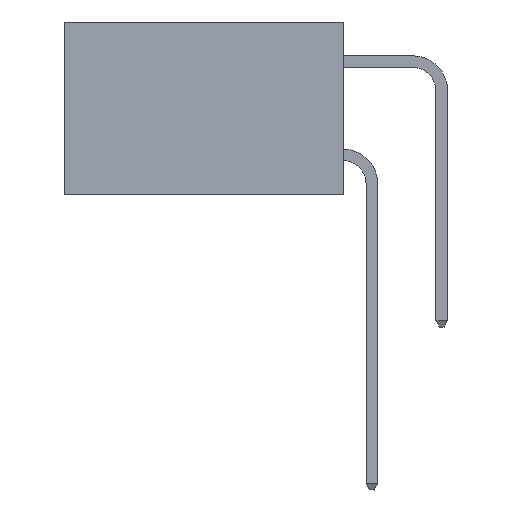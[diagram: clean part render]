
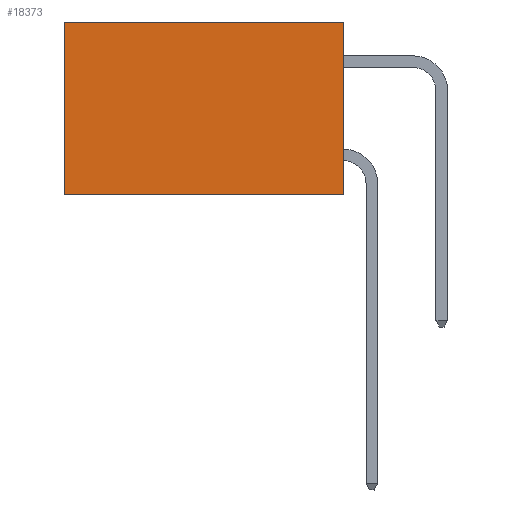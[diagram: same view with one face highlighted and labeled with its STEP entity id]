
A CAD part, left-side view. The second image highlights one B-rep face of the part: STEP entity #18373.
In plain terms, the highlighted planar face has unit normal (-1, 0, 0).
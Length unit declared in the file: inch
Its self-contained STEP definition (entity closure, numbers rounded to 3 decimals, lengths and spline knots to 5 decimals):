
#243 = VERTEX_POINT ( 'NONE', #23693 ) ;
#539 = ORIENTED_EDGE ( 'NONE', *, *, #4084, .T. ) ;
#1354 = LINE ( 'NONE', #24016, #4735 ) ;
#1609 = LINE ( 'NONE', #6266, #12739 ) ;
#3948 = CARTESIAN_POINT ( 'NONE',  ( 0.298, 0.6, 0. ) ) ;
#4084 = EDGE_CURVE ( 'NONE', #29952, #25502, #1609, .T. ) ;
#4362 = DIRECTION ( 'NONE',  ( 0., 0., -1. ) ) ;
#4735 = VECTOR ( 'NONE', #11901, 39.37008 ) ;
#5159 = CARTESIAN_POINT ( 'NONE',  ( 0.298, 0., 0. ) ) ;
#5427 = DIRECTION ( 'NONE',  ( 0., 0., -1. ) ) ;
#5473 = LINE ( 'NONE', #3948, #22225 ) ;
#6266 = CARTESIAN_POINT ( 'NONE',  ( 0.298, 0., 0. ) ) ;
#7708 = CARTESIAN_POINT ( 'NONE',  ( 0.298, 0., -0.37 ) ) ;
#9049 = EDGE_CURVE ( 'NONE', #25502, #29524, #5473, .T. ) ;
#10453 = CARTESIAN_POINT ( 'NONE',  ( 0.298, 0., 0. ) ) ;
#10582 = DIRECTION ( 'NONE',  ( 0., 1., 0. ) ) ;
#11901 = DIRECTION ( 'NONE',  ( 0., 0., -1. ) ) ;
#12660 = LINE ( 'NONE', #7708, #29360 ) ;
#12739 = VECTOR ( 'NONE', #25713, 39.37008 ) ;
#14317 = FACE_OUTER_BOUND ( 'NONE', #17083, .T. ) ;
#16284 = ORIENTED_EDGE ( 'NONE', *, *, #23123, .F. ) ;
#17083 = EDGE_LOOP ( 'NONE', ( #30879, #16284, #17385, #539 ) ) ;
#17385 = ORIENTED_EDGE ( 'NONE', *, *, #18628, .F. ) ;
#18373 = ADVANCED_FACE ( 'NONE', ( #14317 ), #29655, .F. ) ;
#18628 = EDGE_CURVE ( 'NONE', #29952, #243, #1354, .T. ) ;
#18989 = AXIS2_PLACEMENT_3D ( 'NONE', #10453, #25004, #5427 ) ;
#19328 = CARTESIAN_POINT ( 'NONE',  ( 0.298, 0.6, 0. ) ) ;
#22225 = VECTOR ( 'NONE', #4362, 39.37008 ) ;
#22991 = CARTESIAN_POINT ( 'NONE',  ( 0.298, 0.6, -0.37 ) ) ;
#23123 = EDGE_CURVE ( 'NONE', #243, #29524, #12660, .T. ) ;
#23693 = CARTESIAN_POINT ( 'NONE',  ( 0.298, 0., -0.37 ) ) ;
#24016 = CARTESIAN_POINT ( 'NONE',  ( 0.298, 0., 0. ) ) ;
#25004 = DIRECTION ( 'NONE',  ( 1., 0., 0. ) ) ;
#25502 = VERTEX_POINT ( 'NONE', #19328 ) ;
#25713 = DIRECTION ( 'NONE',  ( 0., 1., 0. ) ) ;
#29360 = VECTOR ( 'NONE', #10582, 39.37008 ) ;
#29524 = VERTEX_POINT ( 'NONE', #22991 ) ;
#29655 = PLANE ( 'NONE',  #18989 ) ;
#29952 = VERTEX_POINT ( 'NONE', #5159 ) ;
#30879 = ORIENTED_EDGE ( 'NONE', *, *, #9049, .T. ) ;
